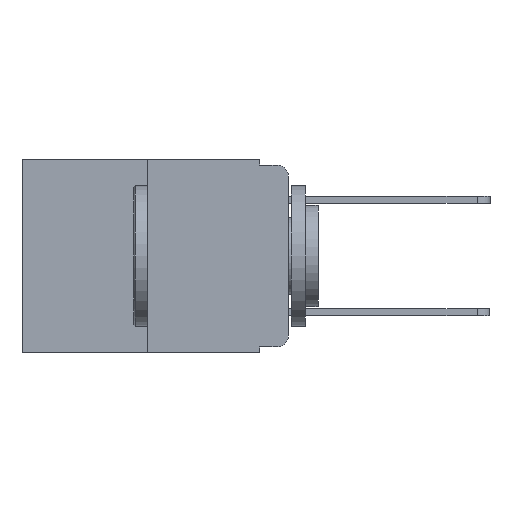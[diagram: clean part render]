
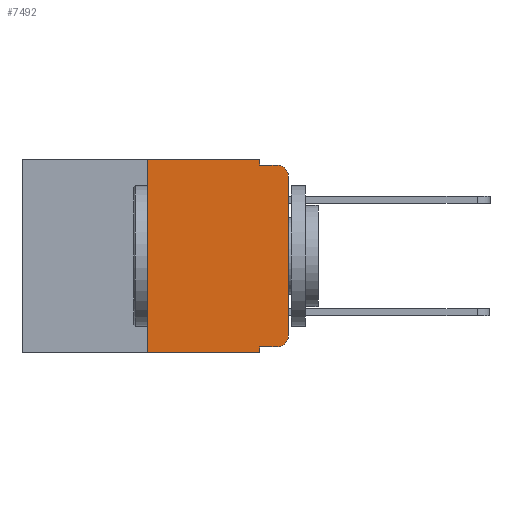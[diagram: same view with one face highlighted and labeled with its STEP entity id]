
A CAD part, left-side view. The second image highlights one B-rep face of the part: STEP entity #7492.
In plain terms, the highlighted planar face has unit normal (-1, 0, 0).
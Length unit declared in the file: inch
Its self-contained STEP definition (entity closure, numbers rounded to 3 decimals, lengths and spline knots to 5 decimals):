
#225 = AXIS2_PLACEMENT_3D ( 'NONE', #25551, #13519, #1102 ) ;
#241 = LINE ( 'NONE', #22159, #10723 ) ;
#388 = CARTESIAN_POINT ( 'NONE',  ( 0., 0.25, 0. ) ) ;
#401 = EDGE_LOOP ( 'NONE', ( #8167, #14170, #25491, #6527, #13236, #25805, #7532, #3907, #21093, #2534 ) ) ;
#990 = PLANE ( 'NONE',  #5622 ) ;
#1102 = DIRECTION ( 'NONE',  ( 0., 0., -1. ) ) ;
#1275 = LINE ( 'NONE', #13909, #11063 ) ;
#2487 = CARTESIAN_POINT ( 'NONE',  ( 0., 0.473, -0.343 ) ) ;
#2534 = ORIENTED_EDGE ( 'NONE', *, *, #22724, .T. ) ;
#2876 = DIRECTION ( 'NONE',  ( 0., 0., 1. ) ) ;
#3067 = EDGE_CURVE ( 'NONE', #11578, #5662, #5764, .T. ) ;
#3138 = CARTESIAN_POINT ( 'NONE',  ( 0., 0.473, 0. ) ) ;
#3173 = EDGE_CURVE ( 'NONE', #13073, #9325, #25985, .T. ) ;
#3266 = CARTESIAN_POINT ( 'NONE',  ( 0., 0.051, -0.333 ) ) ;
#3751 = VECTOR ( 'NONE', #26454, 39.37008 ) ;
#3852 = DIRECTION ( 'NONE',  ( 0., 0., -1. ) ) ;
#3881 = DIRECTION ( 'NONE',  ( 0., 0., 1. ) ) ;
#3894 = CARTESIAN_POINT ( 'NONE',  ( 0., 0.02, -0.313 ) ) ;
#3907 = ORIENTED_EDGE ( 'NONE', *, *, #3067, .F. ) ;
#4636 = VERTEX_POINT ( 'NONE', #25381 ) ;
#5274 = DIRECTION ( 'NONE',  ( 1., 0., 0. ) ) ;
#5622 = AXIS2_PLACEMENT_3D ( 'NONE', #3138, #5274, #19485 ) ;
#5662 = VERTEX_POINT ( 'NONE', #14340 ) ;
#5764 = LINE ( 'NONE', #20094, #16566 ) ;
#5829 = CARTESIAN_POINT ( 'NONE',  ( 0., 0., -0.03 ) ) ;
#5864 = CARTESIAN_POINT ( 'NONE',  ( 0., 0.051, -0.01 ) ) ;
#6038 = DIRECTION ( 'NONE',  ( 0., 0., -1. ) ) ;
#6065 = AXIS2_PLACEMENT_3D ( 'NONE', #3894, #18195, #6038 ) ;
#6527 = ORIENTED_EDGE ( 'NONE', *, *, #10037, .F. ) ;
#7492 = ADVANCED_FACE ( 'NONE', ( #21390 ), #990, .F. ) ;
#7532 = ORIENTED_EDGE ( 'NONE', *, *, #10074, .T. ) ;
#7670 = VERTEX_POINT ( 'NONE', #5829 ) ;
#8167 = ORIENTED_EDGE ( 'NONE', *, *, #17674, .T. ) ;
#8551 = VECTOR ( 'NONE', #22892, 39.37008 ) ;
#8682 = EDGE_CURVE ( 'NONE', #19337, #13073, #25434, .T. ) ;
#9325 = VERTEX_POINT ( 'NONE', #24391 ) ;
#9651 = LINE ( 'NONE', #2487, #15009 ) ;
#10037 = EDGE_CURVE ( 'NONE', #9325, #22689, #10260, .T. ) ;
#10074 = EDGE_CURVE ( 'NONE', #19337, #5662, #9651, .T. ) ;
#10260 = LINE ( 'NONE', #18805, #25690 ) ;
#10723 = VECTOR ( 'NONE', #3881, 39.37008 ) ;
#11063 = VECTOR ( 'NONE', #11899, 39.37008 ) ;
#11498 = CIRCLE ( 'NONE', #225, 0.02 ) ;
#11578 = VERTEX_POINT ( 'NONE', #3266 ) ;
#11899 = DIRECTION ( 'NONE',  ( 0., -1., 0. ) ) ;
#13073 = VERTEX_POINT ( 'NONE', #388 ) ;
#13236 = ORIENTED_EDGE ( 'NONE', *, *, #3173, .F. ) ;
#13519 = DIRECTION ( 'NONE',  ( -1., 0., 0. ) ) ;
#13909 = CARTESIAN_POINT ( 'NONE',  ( 0., 0.051, -0.01 ) ) ;
#14097 = CARTESIAN_POINT ( 'NONE',  ( 0., 0., -0.313 ) ) ;
#14106 = EDGE_CURVE ( 'NONE', #22689, #4636, #1275, .T. ) ;
#14170 = ORIENTED_EDGE ( 'NONE', *, *, #15478, .T. ) ;
#14340 = CARTESIAN_POINT ( 'NONE',  ( 0., 0.051, -0.343 ) ) ;
#14434 = CARTESIAN_POINT ( 'NONE',  ( 0., 0.473, 0. ) ) ;
#14728 = VECTOR ( 'NONE', #2876, 39.37008 ) ;
#15009 = VECTOR ( 'NONE', #22973, 39.37008 ) ;
#15478 = EDGE_CURVE ( 'NONE', #7670, #4636, #11498, .T. ) ;
#16315 = VERTEX_POINT ( 'NONE', #14097 ) ;
#16566 = VECTOR ( 'NONE', #3852, 39.37008 ) ;
#17674 = EDGE_CURVE ( 'NONE', #16315, #7670, #241, .T. ) ;
#18195 = DIRECTION ( 'NONE',  ( -1., 0., 0. ) ) ;
#18805 = CARTESIAN_POINT ( 'NONE',  ( 0., 0.051, 0. ) ) ;
#19337 = VERTEX_POINT ( 'NONE', #19892 ) ;
#19485 = DIRECTION ( 'NONE',  ( 0., 0., -1. ) ) ;
#19892 = CARTESIAN_POINT ( 'NONE',  ( 0., 0.25, -0.343 ) ) ;
#20094 = CARTESIAN_POINT ( 'NONE',  ( 0., 0.051, 0. ) ) ;
#20263 = CIRCLE ( 'NONE', #6065, 0.02 ) ;
#20716 = CARTESIAN_POINT ( 'NONE',  ( 0., 0.02, -0.333 ) ) ;
#20820 = DIRECTION ( 'NONE',  ( 0., 0., -1. ) ) ;
#20824 = CARTESIAN_POINT ( 'NONE',  ( 0., 0.051, -0.333 ) ) ;
#21093 = ORIENTED_EDGE ( 'NONE', *, *, #25397, .T. ) ;
#21200 = CARTESIAN_POINT ( 'NONE',  ( 0., 0.25, 0. ) ) ;
#21390 = FACE_OUTER_BOUND ( 'NONE', #401, .T. ) ;
#22159 = CARTESIAN_POINT ( 'NONE',  ( 0., 0., 0. ) ) ;
#22689 = VERTEX_POINT ( 'NONE', #5864 ) ;
#22724 = EDGE_CURVE ( 'NONE', #22933, #16315, #20263, .T. ) ;
#22892 = DIRECTION ( 'NONE',  ( 0., -1., 0. ) ) ;
#22933 = VERTEX_POINT ( 'NONE', #20716 ) ;
#22973 = DIRECTION ( 'NONE',  ( 0., -1., 0. ) ) ;
#24391 = CARTESIAN_POINT ( 'NONE',  ( 0., 0.051, 0. ) ) ;
#24631 = LINE ( 'NONE', #20824, #8551 ) ;
#25381 = CARTESIAN_POINT ( 'NONE',  ( 0., 0.02, -0.01 ) ) ;
#25397 = EDGE_CURVE ( 'NONE', #11578, #22933, #24631, .T. ) ;
#25434 = LINE ( 'NONE', #21200, #14728 ) ;
#25491 = ORIENTED_EDGE ( 'NONE', *, *, #14106, .F. ) ;
#25551 = CARTESIAN_POINT ( 'NONE',  ( 0., 0.02, -0.03 ) ) ;
#25690 = VECTOR ( 'NONE', #20820, 39.37008 ) ;
#25805 = ORIENTED_EDGE ( 'NONE', *, *, #8682, .F. ) ;
#25985 = LINE ( 'NONE', #14434, #3751 ) ;
#26454 = DIRECTION ( 'NONE',  ( 0., -1., 0. ) ) ;
